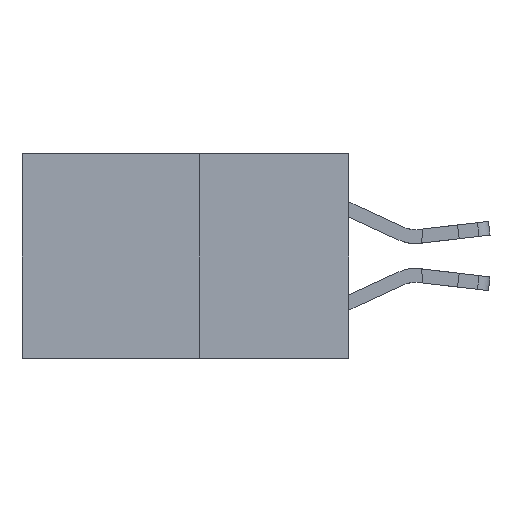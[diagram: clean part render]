
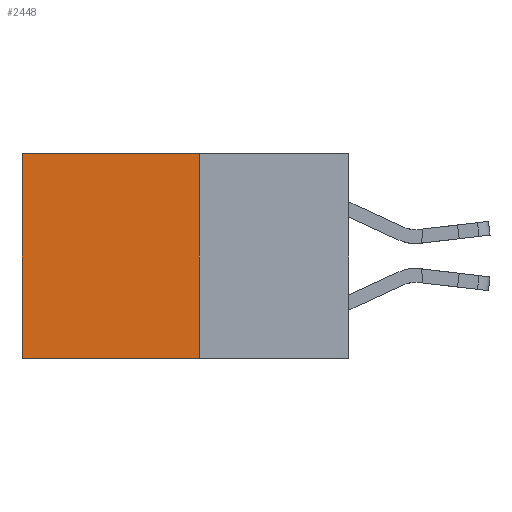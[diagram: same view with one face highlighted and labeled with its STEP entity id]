
A CAD part, left-side view. The second image highlights one B-rep face of the part: STEP entity #2448.
In plain terms, the highlighted planar face has unit normal (-1, 0, 0).
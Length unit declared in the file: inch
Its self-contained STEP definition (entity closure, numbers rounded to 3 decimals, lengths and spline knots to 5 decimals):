
#1174 = ORIENTED_EDGE ( 'NONE', *, *, #6813, .F. ) ;
#1880 = VECTOR ( 'NONE', #5676, 39.37008 ) ;
#1900 = DIRECTION ( 'NONE',  ( 0., 0., -1. ) ) ;
#2448 = ADVANCED_FACE ( 'NONE', ( #5444 ), #16133, .F. ) ;
#2607 = CARTESIAN_POINT ( 'NONE',  ( 0.277, 0.27, 0. ) ) ;
#3201 = EDGE_CURVE ( 'NONE', #3799, #9870, #15026, .T. ) ;
#3502 = CARTESIAN_POINT ( 'NONE',  ( 0.277, 0.27, -0.37 ) ) ;
#3509 = EDGE_LOOP ( 'NONE', ( #12360, #1174, #16322, #17334 ) ) ;
#3799 = VERTEX_POINT ( 'NONE', #7569 ) ;
#3832 = DIRECTION ( 'NONE',  ( 0., 0., -1. ) ) ;
#4092 = LINE ( 'NONE', #14120, #12402 ) ;
#4360 = AXIS2_PLACEMENT_3D ( 'NONE', #9570, #11617, #3832 ) ;
#4728 = CARTESIAN_POINT ( 'NONE',  ( 0.277, 0.27, -0.37 ) ) ;
#5444 = FACE_OUTER_BOUND ( 'NONE', #3509, .T. ) ;
#5676 = DIRECTION ( 'NONE',  ( 0., 0., -1. ) ) ;
#6813 = EDGE_CURVE ( 'NONE', #15023, #9870, #16637, .T. ) ;
#7213 = EDGE_CURVE ( 'NONE', #8641, #3799, #4092, .T. ) ;
#7569 = CARTESIAN_POINT ( 'NONE',  ( 0.277, 0.59, 0. ) ) ;
#8641 = VERTEX_POINT ( 'NONE', #2607 ) ;
#9570 = CARTESIAN_POINT ( 'NONE',  ( 0.277, 0.27, -0.37 ) ) ;
#9870 = VERTEX_POINT ( 'NONE', #20195 ) ;
#9962 = LINE ( 'NONE', #11875, #19523 ) ;
#11617 = DIRECTION ( 'NONE',  ( 1., 0., 0. ) ) ;
#11836 = CARTESIAN_POINT ( 'NONE',  ( 0.277, 0.59, -0.37 ) ) ;
#11875 = CARTESIAN_POINT ( 'NONE',  ( 0.277, 0.27, -0.37 ) ) ;
#12126 = DIRECTION ( 'NONE',  ( 0., 1., 0. ) ) ;
#12360 = ORIENTED_EDGE ( 'NONE', *, *, #3201, .T. ) ;
#12402 = VECTOR ( 'NONE', #13710, 39.37008 ) ;
#13710 = DIRECTION ( 'NONE',  ( 0., 1., 0. ) ) ;
#14120 = CARTESIAN_POINT ( 'NONE',  ( 0.277, 0.27, 0. ) ) ;
#15023 = VERTEX_POINT ( 'NONE', #3502 ) ;
#15026 = LINE ( 'NONE', #11836, #1880 ) ;
#16133 = PLANE ( 'NONE',  #4360 ) ;
#16322 = ORIENTED_EDGE ( 'NONE', *, *, #16917, .F. ) ;
#16637 = LINE ( 'NONE', #4728, #20845 ) ;
#16917 = EDGE_CURVE ( 'NONE', #8641, #15023, #9962, .T. ) ;
#17334 = ORIENTED_EDGE ( 'NONE', *, *, #7213, .T. ) ;
#19523 = VECTOR ( 'NONE', #1900, 39.37008 ) ;
#20195 = CARTESIAN_POINT ( 'NONE',  ( 0.277, 0.59, -0.37 ) ) ;
#20845 = VECTOR ( 'NONE', #12126, 39.37008 ) ;
